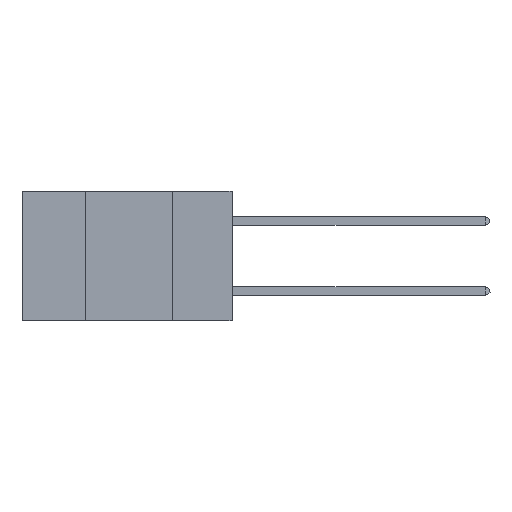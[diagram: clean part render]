
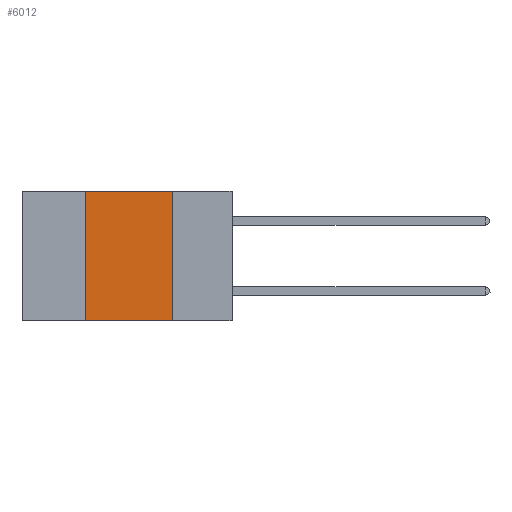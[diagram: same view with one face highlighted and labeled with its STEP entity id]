
A CAD part, left-side view. The second image highlights one B-rep face of the part: STEP entity #6012.
In plain terms, the highlighted planar face has unit normal (-1, 0, 0).
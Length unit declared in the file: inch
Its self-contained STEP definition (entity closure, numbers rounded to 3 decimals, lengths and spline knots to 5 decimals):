
#206 = DIRECTION ( 'NONE',  ( 0., 0., -1. ) ) ;
#286 = VECTOR ( 'NONE', #2686, 39.37008 ) ;
#1287 = CARTESIAN_POINT ( 'NONE',  ( 0., 0.42, 0. ) ) ;
#1418 = ORIENTED_EDGE ( 'NONE', *, *, #8252, .F. ) ;
#1790 = CARTESIAN_POINT ( 'NONE',  ( 0., 0.17, 0. ) ) ;
#2209 = EDGE_LOOP ( 'NONE', ( #1418, #5839, #10381, #6639 ) ) ;
#2254 = DIRECTION ( 'NONE',  ( 0., 0., 1. ) ) ;
#2686 = DIRECTION ( 'NONE',  ( 0., -1., 0. ) ) ;
#2832 = CARTESIAN_POINT ( 'NONE',  ( 0., 0.17, 0. ) ) ;
#3672 = DIRECTION ( 'NONE',  ( 1., 0., 0. ) ) ;
#3778 = CARTESIAN_POINT ( 'NONE',  ( 0., 0.42, -0.37 ) ) ;
#4009 = DIRECTION ( 'NONE',  ( 0., 0., -1. ) ) ;
#4279 = CARTESIAN_POINT ( 'NONE',  ( 0., 0.42, 0. ) ) ;
#4791 = FACE_OUTER_BOUND ( 'NONE', #2209, .T. ) ;
#5057 = LINE ( 'NONE', #2832, #14327 ) ;
#5839 = ORIENTED_EDGE ( 'NONE', *, *, #7525, .F. ) ;
#6012 = ADVANCED_FACE ( 'NONE', ( #4791 ), #6823, .F. ) ;
#6148 = CARTESIAN_POINT ( 'NONE',  ( 0., 0.17, -0.37 ) ) ;
#6639 = ORIENTED_EDGE ( 'NONE', *, *, #8766, .T. ) ;
#6823 = PLANE ( 'NONE',  #9187 ) ;
#7078 = CARTESIAN_POINT ( 'NONE',  ( 0., 0.6, -0.37 ) ) ;
#7525 = EDGE_CURVE ( 'NONE', #11613, #8330, #9863, .T. ) ;
#7554 = VECTOR ( 'NONE', #2254, 39.37008 ) ;
#8150 = EDGE_CURVE ( 'NONE', #14161, #11613, #13382, .T. ) ;
#8252 = EDGE_CURVE ( 'NONE', #8330, #13873, #5057, .T. ) ;
#8330 = VERTEX_POINT ( 'NONE', #1790 ) ;
#8687 = DIRECTION ( 'NONE',  ( 0., -1., 0. ) ) ;
#8763 = CARTESIAN_POINT ( 'NONE',  ( 0., 0.6, 0. ) ) ;
#8766 = EDGE_CURVE ( 'NONE', #14161, #13873, #12709, .T. ) ;
#9187 = AXIS2_PLACEMENT_3D ( 'NONE', #13708, #3672, #206 ) ;
#9863 = LINE ( 'NONE', #8763, #12200 ) ;
#10381 = ORIENTED_EDGE ( 'NONE', *, *, #8150, .F. ) ;
#11613 = VERTEX_POINT ( 'NONE', #4279 ) ;
#12200 = VECTOR ( 'NONE', #8687, 39.37008 ) ;
#12709 = LINE ( 'NONE', #7078, #286 ) ;
#13382 = LINE ( 'NONE', #1287, #7554 ) ;
#13708 = CARTESIAN_POINT ( 'NONE',  ( 0., 0.6, 0. ) ) ;
#13873 = VERTEX_POINT ( 'NONE', #6148 ) ;
#14161 = VERTEX_POINT ( 'NONE', #3778 ) ;
#14327 = VECTOR ( 'NONE', #4009, 39.37008 ) ;
